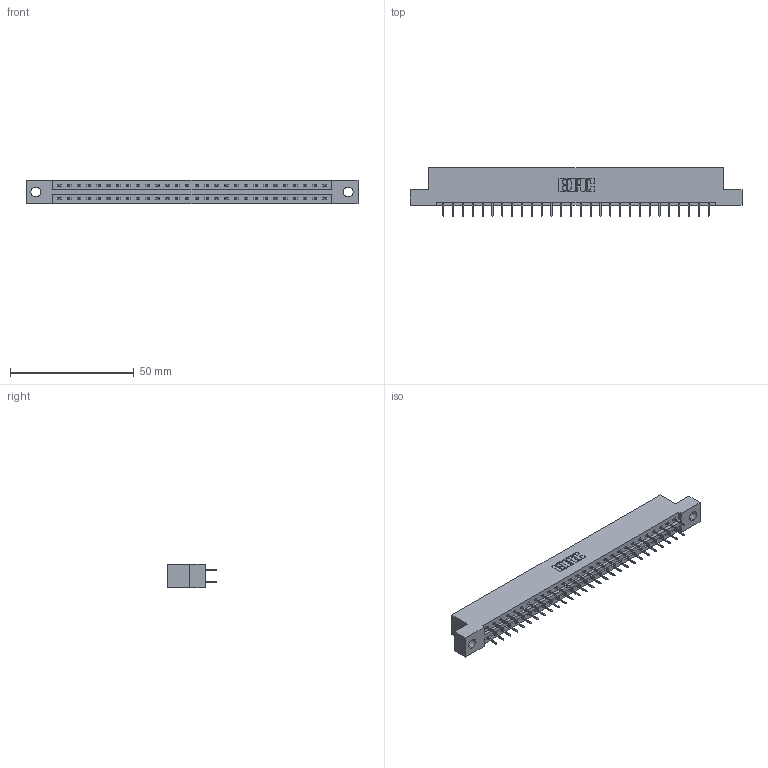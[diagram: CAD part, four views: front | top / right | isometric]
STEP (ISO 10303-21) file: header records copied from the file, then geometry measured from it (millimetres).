
FILE_DESCRIPTION (( 'STEP AP203' ), '1' );
FILE_NAME ('337-056-524-204.STEP', '2019-10-09T18:55:47', ( '' ), ( '' ), 'SwSTEP 2.0', 'SolidWorks 2016', '' );
FILE_SCHEMA (( 'CONFIG_CONTROL_DESIGN' ));
Length unit declared in the file: inch
Products named in the file (3): 337 Part_Flush Mounting Lugs - 0.156 Dia-TH; 345-292-001_345-293-124; 337-056-524-204
Assembly tree (57 placements, depth 2):
  337-056-524-204
    337 Part_Flush Mounting Lugs - 0.156 Dia-TH
    345-292-001_345-293-124  x56
Bounding box: 133.96 x 19.69 x 9.4 mm (x, y, z)
Volume: 13758.8 mm3; surface area: 14953.2 mm2
Topology: 57 solids, 57 shells, 3362 faces, 9551 edges, 6142 vertices
Faces by surface type: plane 2534, cylinder 828
Entity records: 23597 total; most frequent: CARTESIAN_POINT 3986, ORIENTED_EDGE 3922, DIRECTION 3417, EDGE_CURVE 1961, LINE 1837, VECTOR 1837, VERTEX_POINT 1302, AXIS2_PLACEMENT_3D 790
